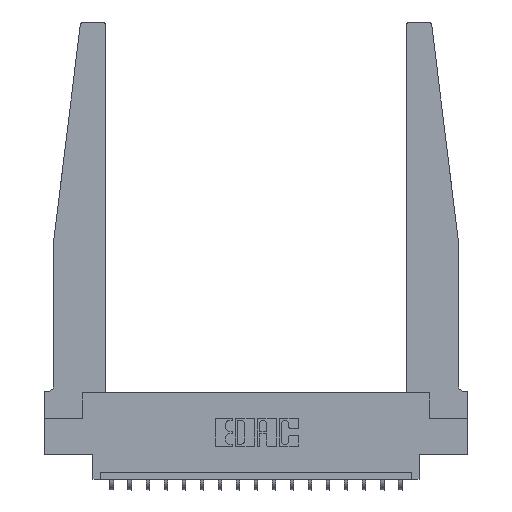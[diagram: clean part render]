
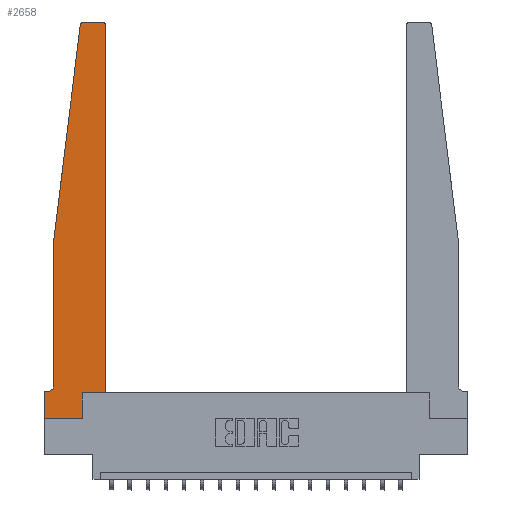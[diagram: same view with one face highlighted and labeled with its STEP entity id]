
A CAD part, top view. The second image highlights one B-rep face of the part: STEP entity #2658.
In plain terms, the highlighted planar face has unit normal (0, 0, 1).
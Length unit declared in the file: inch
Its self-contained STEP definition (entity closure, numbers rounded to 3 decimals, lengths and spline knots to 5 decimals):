
#115 = CARTESIAN_POINT ( 'NONE',  ( 0.425, 0.18, 0.37 ) ) ;
#213 = CIRCLE ( 'NONE', #11171, 0.03 ) ;
#547 = ORIENTED_EDGE ( 'NONE', *, *, #2096, .T. ) ;
#552 = CARTESIAN_POINT ( 'NONE',  ( 0.065, 0.1875, 0.37 ) ) ;
#638 = LINE ( 'NONE', #6631, #10046 ) ;
#642 = LINE ( 'NONE', #552, #13413 ) ;
#832 = CARTESIAN_POINT ( 'NONE',  ( 0., 0., 0.37 ) ) ;
#1164 = VERTEX_POINT ( 'NONE', #3136 ) ;
#1337 = CARTESIAN_POINT ( 'NONE',  ( 0.065, 1.25, 0.37 ) ) ;
#1398 = CARTESIAN_POINT ( 'NONE',  ( 0.065, 1.25, 0.37 ) ) ;
#1438 = DIRECTION ( 'NONE',  ( 0., 0., 1. ) ) ;
#1496 = LINE ( 'NONE', #1690, #17698 ) ;
#1690 = CARTESIAN_POINT ( 'NONE',  ( 0.425, 0.18, 0.37 ) ) ;
#1845 = CARTESIAN_POINT ( 'NONE',  ( 0.065, 0.2375, 0.37 ) ) ;
#2096 = EDGE_CURVE ( 'NONE', #14969, #3192, #213, .T. ) ;
#2199 = DIRECTION ( 'NONE',  ( 0., 0., 1. ) ) ;
#2225 = VECTOR ( 'NONE', #14152, 39.37008 ) ;
#2337 = ORIENTED_EDGE ( 'NONE', *, *, #4983, .T. ) ;
#2496 = VERTEX_POINT ( 'NONE', #2872 ) ;
#2523 = CARTESIAN_POINT ( 'NONE',  ( 0.24675, 2.72367, 0.37 ) ) ;
#2658 = ADVANCED_FACE ( 'NONE', ( #2737 ), #8900, .T. ) ;
#2737 = FACE_OUTER_BOUND ( 'NONE', #6604, .T. ) ;
#2765 = AXIS2_PLACEMENT_3D ( 'NONE', #7224, #1438, #17144 ) ;
#2815 = EDGE_CURVE ( 'NONE', #19195, #1164, #16493, .T. ) ;
#2872 = CARTESIAN_POINT ( 'NONE',  ( 0.425, 2.72, 0.37 ) ) ;
#3120 = EDGE_CURVE ( 'NONE', #1164, #16270, #642, .T. ) ;
#3136 = CARTESIAN_POINT ( 'NONE',  ( 0.015, 0.1875, 0.37 ) ) ;
#3192 = VERTEX_POINT ( 'NONE', #2523 ) ;
#3411 = DIRECTION ( 'NONE',  ( 0., 0., -1. ) ) ;
#3447 = ORIENTED_EDGE ( 'NONE', *, *, #8704, .T. ) ;
#3668 = DIRECTION ( 'NONE',  ( 1., 0., 0. ) ) ;
#3925 = EDGE_CURVE ( 'NONE', #16270, #16822, #4735, .T. ) ;
#3978 = CIRCLE ( 'NONE', #10557, 0.03 ) ;
#4513 = EDGE_CURVE ( 'NONE', #7238, #5194, #638, .T. ) ;
#4735 = LINE ( 'NONE', #16671, #10953 ) ;
#4983 = EDGE_CURVE ( 'NONE', #11988, #14969, #14443, .T. ) ;
#4985 = DIRECTION ( 'NONE',  ( 1., 0., 0. ) ) ;
#4993 = ORIENTED_EDGE ( 'NONE', *, *, #12912, .T. ) ;
#5104 = ORIENTED_EDGE ( 'NONE', *, *, #4513, .T. ) ;
#5194 = VERTEX_POINT ( 'NONE', #13253 ) ;
#5341 = EDGE_CURVE ( 'NONE', #2496, #11988, #3978, .T. ) ;
#5891 = CARTESIAN_POINT ( 'NONE',  ( 0.065, 1.25, 0.37 ) ) ;
#5933 = LINE ( 'NONE', #11903, #8363 ) ;
#5962 = DIRECTION ( 'NONE',  ( 0., -1., 0. ) ) ;
#6027 = DIRECTION ( 'NONE',  ( 0., 1., 0. ) ) ;
#6344 = DIRECTION ( 'NONE',  ( 0., 1., 0. ) ) ;
#6372 = CARTESIAN_POINT ( 'NONE',  ( 0.395, 2.75, 0.37 ) ) ;
#6604 = EDGE_LOOP ( 'NONE', ( #2337, #547, #3447, #16663, #8729, #14734, #13768, #14528, #5104, #14414, #4993, #11670 ) ) ;
#6631 = CARTESIAN_POINT ( 'NONE',  ( 0.2605, 0.18, 0.37 ) ) ;
#7196 = CARTESIAN_POINT ( 'NONE',  ( 0.2605, 0., 0.37 ) ) ;
#7224 = CARTESIAN_POINT ( 'NONE',  ( 0., 0.1875, 0.37 ) ) ;
#7238 = VERTEX_POINT ( 'NONE', #7196 ) ;
#7471 = DIRECTION ( 'NONE',  ( 1., 0., 0. ) ) ;
#7631 = VECTOR ( 'NONE', #5962, 39.37008 ) ;
#7756 = CARTESIAN_POINT ( 'NONE',  ( 0., 0.1875, 0.37 ) ) ;
#8267 = EDGE_CURVE ( 'NONE', #5194, #16244, #1496, .T. ) ;
#8353 = DIRECTION ( 'NONE',  ( 0., 0., 1. ) ) ;
#8363 = VECTOR ( 'NONE', #6027, 39.37008 ) ;
#8704 = EDGE_CURVE ( 'NONE', #3192, #9534, #15194, .T. ) ;
#8729 = ORIENTED_EDGE ( 'NONE', *, *, #2815, .T. ) ;
#8900 = PLANE ( 'NONE',  #2765 ) ;
#9401 = CARTESIAN_POINT ( 'NONE',  ( 0., 0., 0.37 ) ) ;
#9485 = DIRECTION ( 'NONE',  ( -1., 0., 0. ) ) ;
#9534 = VERTEX_POINT ( 'NONE', #1398 ) ;
#10046 = VECTOR ( 'NONE', #6344, 39.37008 ) ;
#10216 = VECTOR ( 'NONE', #12159, 39.37008 ) ;
#10346 = EDGE_CURVE ( 'NONE', #9534, #19195, #12231, .T. ) ;
#10557 = AXIS2_PLACEMENT_3D ( 'NONE', #15779, #8353, #17145 ) ;
#10750 = CARTESIAN_POINT ( 'NONE',  ( 0.015, 0.2375, 0.37 ) ) ;
#10953 = VECTOR ( 'NONE', #13568, 39.37008 ) ;
#11171 = AXIS2_PLACEMENT_3D ( 'NONE', #15235, #2199, #3668 ) ;
#11670 = ORIENTED_EDGE ( 'NONE', *, *, #5341, .T. ) ;
#11903 = CARTESIAN_POINT ( 'NONE',  ( 0.425, 0.18, 0.37 ) ) ;
#11988 = VERTEX_POINT ( 'NONE', #6372 ) ;
#12159 = DIRECTION ( 'NONE',  ( -0.122, -0.992, 0. ) ) ;
#12231 = LINE ( 'NONE', #1337, #7631 ) ;
#12434 = LINE ( 'NONE', #9401, #15965 ) ;
#12769 = AXIS2_PLACEMENT_3D ( 'NONE', #10750, #3411, #16812 ) ;
#12912 = EDGE_CURVE ( 'NONE', #16244, #2496, #5933, .T. ) ;
#13253 = CARTESIAN_POINT ( 'NONE',  ( 0.2605, 0.18, 0.37 ) ) ;
#13413 = VECTOR ( 'NONE', #9485, 39.37008 ) ;
#13441 = CARTESIAN_POINT ( 'NONE',  ( 0.27653, 2.75, 0.37 ) ) ;
#13568 = DIRECTION ( 'NONE',  ( 0., -1., 0. ) ) ;
#13768 = ORIENTED_EDGE ( 'NONE', *, *, #3925, .T. ) ;
#14152 = DIRECTION ( 'NONE',  ( -1., 0., 0. ) ) ;
#14414 = ORIENTED_EDGE ( 'NONE', *, *, #8267, .T. ) ;
#14443 = LINE ( 'NONE', #17451, #2225 ) ;
#14528 = ORIENTED_EDGE ( 'NONE', *, *, #19162, .T. ) ;
#14734 = ORIENTED_EDGE ( 'NONE', *, *, #3120, .T. ) ;
#14969 = VERTEX_POINT ( 'NONE', #13441 ) ;
#15194 = LINE ( 'NONE', #5891, #10216 ) ;
#15235 = CARTESIAN_POINT ( 'NONE',  ( 0.27653, 2.72, 0.37 ) ) ;
#15779 = CARTESIAN_POINT ( 'NONE',  ( 0.395, 2.72, 0.37 ) ) ;
#15965 = VECTOR ( 'NONE', #4985, 39.37008 ) ;
#16244 = VERTEX_POINT ( 'NONE', #115 ) ;
#16270 = VERTEX_POINT ( 'NONE', #7756 ) ;
#16493 = CIRCLE ( 'NONE', #12769, 0.05 ) ;
#16663 = ORIENTED_EDGE ( 'NONE', *, *, #10346, .T. ) ;
#16671 = CARTESIAN_POINT ( 'NONE',  ( 0., 0., 0.37 ) ) ;
#16812 = DIRECTION ( 'NONE',  ( -1., 0., 0. ) ) ;
#16822 = VERTEX_POINT ( 'NONE', #832 ) ;
#17144 = DIRECTION ( 'NONE',  ( 1., 0., 0. ) ) ;
#17145 = DIRECTION ( 'NONE',  ( 1., 0., 0. ) ) ;
#17451 = CARTESIAN_POINT ( 'NONE',  ( 0.25, 2.75, 0.37 ) ) ;
#17698 = VECTOR ( 'NONE', #7471, 39.37008 ) ;
#19162 = EDGE_CURVE ( 'NONE', #16822, #7238, #12434, .T. ) ;
#19195 = VERTEX_POINT ( 'NONE', #1845 ) ;
